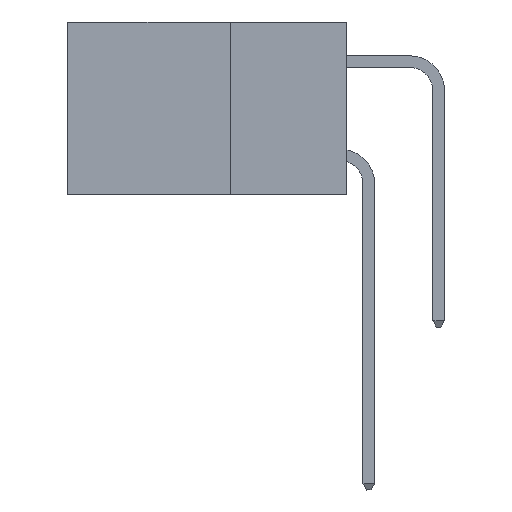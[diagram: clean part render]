
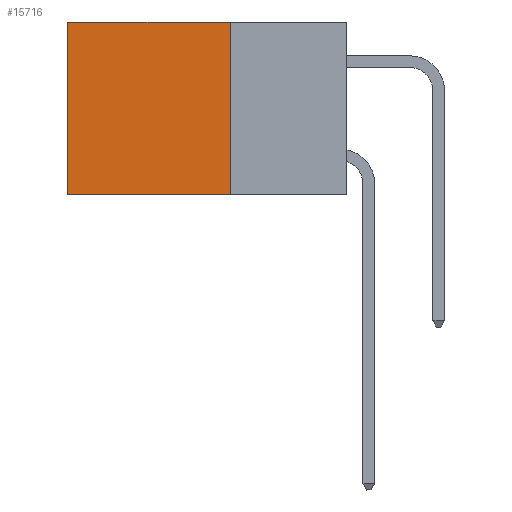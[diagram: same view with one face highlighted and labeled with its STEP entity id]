
A CAD part, left-side view. The second image highlights one B-rep face of the part: STEP entity #15716.
In plain terms, the highlighted planar face has unit normal (-1, 0, 0).
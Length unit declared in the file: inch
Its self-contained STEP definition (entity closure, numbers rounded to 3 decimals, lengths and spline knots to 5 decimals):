
#242 = CARTESIAN_POINT ( 'NONE',  ( 0.2875, 0.6, -0.37 ) ) ;
#536 = FACE_OUTER_BOUND ( 'NONE', #12945, .T. ) ;
#568 = DIRECTION ( 'NONE',  ( 1., 0., 0. ) ) ;
#646 = DIRECTION ( 'NONE',  ( 0., 1., 0. ) ) ;
#2536 = DIRECTION ( 'NONE',  ( 0., 0., -1. ) ) ;
#3030 = CARTESIAN_POINT ( 'NONE',  ( 0.2875, 0.25, -0.37 ) ) ;
#4225 = CARTESIAN_POINT ( 'NONE',  ( 0.2875, 0.25, 0. ) ) ;
#5235 = CARTESIAN_POINT ( 'NONE',  ( 0.2875, 0.6, 0. ) ) ;
#7106 = VECTOR ( 'NONE', #17689, 39.37008 ) ;
#8518 = ORIENTED_EDGE ( 'NONE', *, *, #17136, .T. ) ;
#9291 = LINE ( 'NONE', #16837, #12308 ) ;
#9353 = VECTOR ( 'NONE', #16879, 39.37008 ) ;
#10947 = EDGE_CURVE ( 'NONE', #19410, #13232, #18753, .T. ) ;
#12308 = VECTOR ( 'NONE', #15798, 39.37008 ) ;
#12360 = AXIS2_PLACEMENT_3D ( 'NONE', #20097, #568, #2536 ) ;
#12917 = CARTESIAN_POINT ( 'NONE',  ( 0.2875, 0.25, -0.37 ) ) ;
#12945 = EDGE_LOOP ( 'NONE', ( #8518, #16581, #18071, #19722 ) ) ;
#13232 = VERTEX_POINT ( 'NONE', #242 ) ;
#15716 = ADVANCED_FACE ( 'NONE', ( #536 ), #21800, .F. ) ;
#15798 = DIRECTION ( 'NONE',  ( 0., 0., -1. ) ) ;
#16581 = ORIENTED_EDGE ( 'NONE', *, *, #10947, .F. ) ;
#16721 = LINE ( 'NONE', #21305, #7106 ) ;
#16837 = CARTESIAN_POINT ( 'NONE',  ( 0.2875, 0.6, 0. ) ) ;
#16879 = DIRECTION ( 'NONE',  ( 0., 1., 0. ) ) ;
#17136 = EDGE_CURVE ( 'NONE', #18087, #13232, #9291, .T. ) ;
#17512 = EDGE_CURVE ( 'NONE', #21931, #19410, #16721, .T. ) ;
#17689 = DIRECTION ( 'NONE',  ( 0., 0., -1. ) ) ;
#18071 = ORIENTED_EDGE ( 'NONE', *, *, #17512, .F. ) ;
#18087 = VERTEX_POINT ( 'NONE', #5235 ) ;
#18697 = CARTESIAN_POINT ( 'NONE',  ( 0.2875, 0.25, 0. ) ) ;
#18753 = LINE ( 'NONE', #12917, #9353 ) ;
#18789 = LINE ( 'NONE', #4225, #20130 ) ;
#19410 = VERTEX_POINT ( 'NONE', #3030 ) ;
#19722 = ORIENTED_EDGE ( 'NONE', *, *, #21782, .T. ) ;
#20097 = CARTESIAN_POINT ( 'NONE',  ( 0.2875, 0.25, 0. ) ) ;
#20130 = VECTOR ( 'NONE', #646, 39.37008 ) ;
#21305 = CARTESIAN_POINT ( 'NONE',  ( 0.2875, 0.25, 0. ) ) ;
#21782 = EDGE_CURVE ( 'NONE', #21931, #18087, #18789, .T. ) ;
#21800 = PLANE ( 'NONE',  #12360 ) ;
#21931 = VERTEX_POINT ( 'NONE', #18697 ) ;
